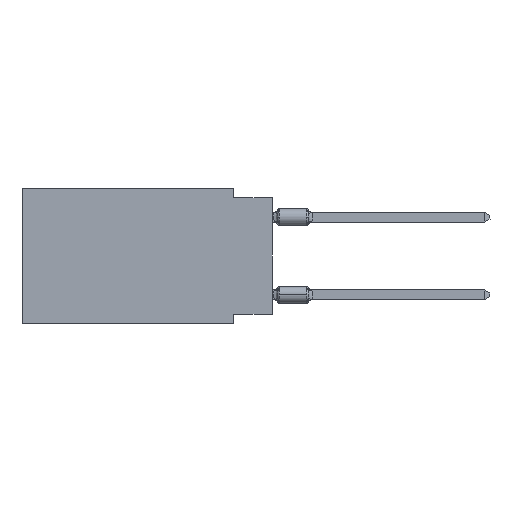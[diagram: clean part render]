
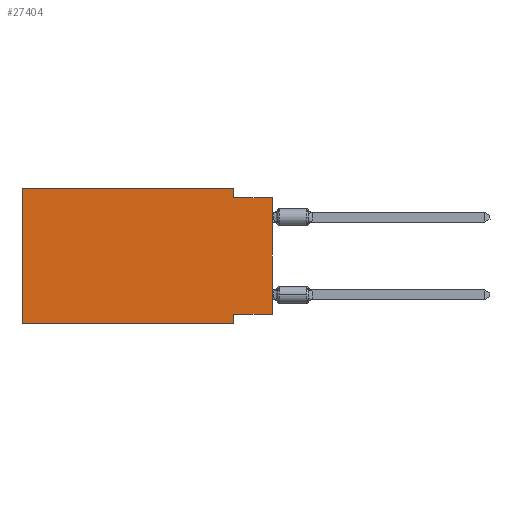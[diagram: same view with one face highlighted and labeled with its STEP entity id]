
A CAD part, left-side view. The second image highlights one B-rep face of the part: STEP entity #27404.
In plain terms, the highlighted planar face has unit normal (-1, 0, 0).
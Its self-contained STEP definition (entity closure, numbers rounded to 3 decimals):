
#489 = AXIS2_PLACEMENT_3D ( 'NONE', #16574, #906, #4997 ) ;
#906 = DIRECTION ( 'NONE',  ( 1., 0., 0. ) ) ;
#922 = CARTESIAN_POINT ( 'NONE',  ( 0., 2.54, -8.89 ) ) ;
#1209 = DIRECTION ( 'NONE',  ( 0., -1., 0. ) ) ;
#1458 = EDGE_CURVE ( 'NONE', #17656, #4338, #6046, .T. ) ;
#1754 = LINE ( 'NONE', #26213, #7467 ) ;
#2143 = EDGE_LOOP ( 'NONE', ( #19187, #24142, #8272, #18548, #24544, #5070, #14326, #13211 ) ) ;
#2631 = CARTESIAN_POINT ( 'NONE',  ( 0., 16.383, 0. ) ) ;
#2795 = CARTESIAN_POINT ( 'NONE',  ( 0., 2.54, 0. ) ) ;
#2929 = VERTEX_POINT ( 'NONE', #922 ) ;
#3844 = DIRECTION ( 'NONE',  ( 0., 0., 1. ) ) ;
#4318 = VECTOR ( 'NONE', #12090, 1000. ) ;
#4338 = VERTEX_POINT ( 'NONE', #11582 ) ;
#4997 = DIRECTION ( 'NONE',  ( 0., 0., -1. ) ) ;
#5070 = ORIENTED_EDGE ( 'NONE', *, *, #14883, .T. ) ;
#5995 = CARTESIAN_POINT ( 'NONE',  ( 0., 2.54, -0.635 ) ) ;
#6046 = LINE ( 'NONE', #25982, #13866 ) ;
#7467 = VECTOR ( 'NONE', #21836, 1000. ) ;
#7935 = CARTESIAN_POINT ( 'NONE',  ( 0., 16.383, -8.89 ) ) ;
#7982 = CARTESIAN_POINT ( 'NONE',  ( 0., 0., -0.635 ) ) ;
#8245 = CARTESIAN_POINT ( 'NONE',  ( 0., 0., -8.255 ) ) ;
#8254 = VERTEX_POINT ( 'NONE', #19782 ) ;
#8272 = ORIENTED_EDGE ( 'NONE', *, *, #26452, .F. ) ;
#8372 = VECTOR ( 'NONE', #17999, 1000. ) ;
#9868 = LINE ( 'NONE', #12527, #4318 ) ;
#10982 = DIRECTION ( 'NONE',  ( 0., -1., 0. ) ) ;
#11163 = CARTESIAN_POINT ( 'NONE',  ( 0., 0., -8.255 ) ) ;
#11582 = CARTESIAN_POINT ( 'NONE',  ( 0., 16.383, 0. ) ) ;
#11746 = PLANE ( 'NONE',  #489 ) ;
#12090 = DIRECTION ( 'NONE',  ( 0., 0., 1. ) ) ;
#12463 = VECTOR ( 'NONE', #25576, 1000. ) ;
#12527 = CARTESIAN_POINT ( 'NONE',  ( 0., 0., 0. ) ) ;
#13211 = ORIENTED_EDGE ( 'NONE', *, *, #19861, .F. ) ;
#13494 = LINE ( 'NONE', #2631, #17496 ) ;
#13519 = LINE ( 'NONE', #11163, #27692 ) ;
#13866 = VECTOR ( 'NONE', #3844, 1000. ) ;
#13882 = CARTESIAN_POINT ( 'NONE',  ( 0., 0., -0.635 ) ) ;
#14326 = ORIENTED_EDGE ( 'NONE', *, *, #26306, .F. ) ;
#14883 = EDGE_CURVE ( 'NONE', #17656, #2929, #27583, .T. ) ;
#15284 = DIRECTION ( 'NONE',  ( 0., 1., 0. ) ) ;
#16574 = CARTESIAN_POINT ( 'NONE',  ( 0., 16.383, 0. ) ) ;
#17453 = EDGE_CURVE ( 'NONE', #18800, #18121, #9868, .T. ) ;
#17496 = VECTOR ( 'NONE', #10982, 1000. ) ;
#17656 = VERTEX_POINT ( 'NONE', #21732 ) ;
#17999 = DIRECTION ( 'NONE',  ( 0., 0., -1. ) ) ;
#18121 = VERTEX_POINT ( 'NONE', #13882 ) ;
#18476 = FACE_OUTER_BOUND ( 'NONE', #2143, .T. ) ;
#18548 = ORIENTED_EDGE ( 'NONE', *, *, #19342, .F. ) ;
#18800 = VERTEX_POINT ( 'NONE', #8245 ) ;
#19187 = ORIENTED_EDGE ( 'NONE', *, *, #17453, .T. ) ;
#19342 = EDGE_CURVE ( 'NONE', #4338, #20529, #13494, .T. ) ;
#19782 = CARTESIAN_POINT ( 'NONE',  ( 0., 2.54, -8.255 ) ) ;
#19861 = EDGE_CURVE ( 'NONE', #18800, #8254, #13519, .T. ) ;
#20055 = CARTESIAN_POINT ( 'NONE',  ( 0., 2.54, 0. ) ) ;
#20529 = VERTEX_POINT ( 'NONE', #2795 ) ;
#20650 = VERTEX_POINT ( 'NONE', #5995 ) ;
#21732 = CARTESIAN_POINT ( 'NONE',  ( 0., 16.383, -8.89 ) ) ;
#21836 = DIRECTION ( 'NONE',  ( 0., 0., -1. ) ) ;
#22771 = EDGE_CURVE ( 'NONE', #20650, #18121, #27926, .T. ) ;
#24142 = ORIENTED_EDGE ( 'NONE', *, *, #22771, .F. ) ;
#24544 = ORIENTED_EDGE ( 'NONE', *, *, #1458, .F. ) ;
#24744 = LINE ( 'NONE', #20055, #8372 ) ;
#25391 = VECTOR ( 'NONE', #1209, 1000. ) ;
#25576 = DIRECTION ( 'NONE',  ( 0., -1., 0. ) ) ;
#25982 = CARTESIAN_POINT ( 'NONE',  ( 0., 16.383, 0. ) ) ;
#26213 = CARTESIAN_POINT ( 'NONE',  ( 0., 2.54, -8.89 ) ) ;
#26306 = EDGE_CURVE ( 'NONE', #8254, #2929, #1754, .T. ) ;
#26452 = EDGE_CURVE ( 'NONE', #20529, #20650, #24744, .T. ) ;
#27404 = ADVANCED_FACE ( 'NONE', ( #18476 ), #11746, .F. ) ;
#27583 = LINE ( 'NONE', #7935, #25391 ) ;
#27692 = VECTOR ( 'NONE', #15284, 1000. ) ;
#27926 = LINE ( 'NONE', #7982, #12463 ) ;
